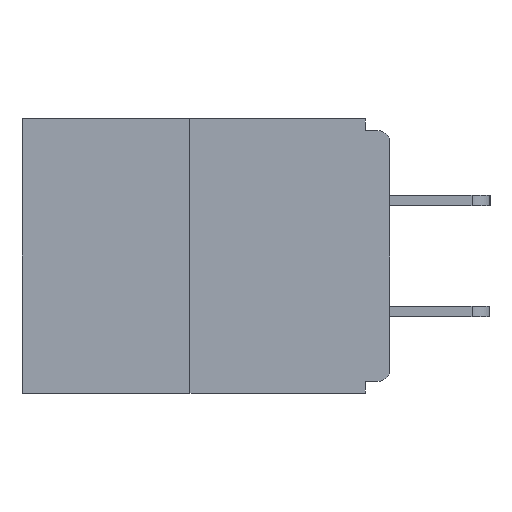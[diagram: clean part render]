
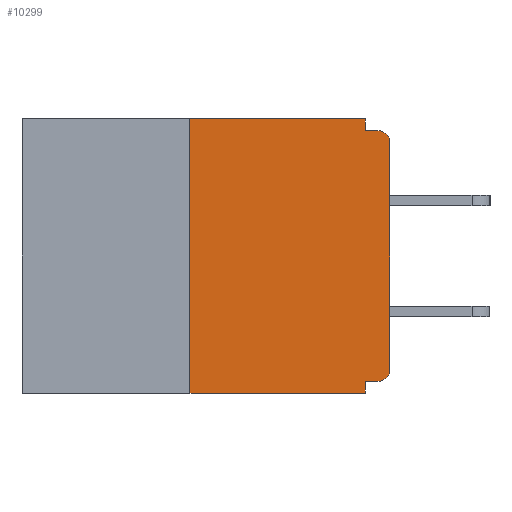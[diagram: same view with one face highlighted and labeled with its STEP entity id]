
A CAD part, left-side view. The second image highlights one B-rep face of the part: STEP entity #10299.
In plain terms, the highlighted planar face has unit normal (-1, 0, 0).
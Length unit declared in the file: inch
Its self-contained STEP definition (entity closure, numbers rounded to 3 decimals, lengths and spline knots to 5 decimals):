
#517 = LINE ( 'NONE', #9732, #7745 ) ;
#551 = VERTEX_POINT ( 'NONE', #4970 ) ;
#664 = EDGE_CURVE ( 'NONE', #4045, #1110, #4424, .T. ) ;
#794 = VERTEX_POINT ( 'NONE', #8882 ) ;
#1110 = VERTEX_POINT ( 'NONE', #6751 ) ;
#1453 = DIRECTION ( 'NONE',  ( 0., 0., -1. ) ) ;
#1519 = EDGE_LOOP ( 'NONE', ( #9037, #9609, #8001, #7870, #8754, #4073, #1643, #8099, #3055, #11710 ) ) ;
#1613 = VECTOR ( 'NONE', #11980, 39.37008 ) ;
#1643 = ORIENTED_EDGE ( 'NONE', *, *, #7530, .T. ) ;
#1729 = CARTESIAN_POINT ( 'NONE',  ( 0., 0., -0.328 ) ) ;
#1971 = EDGE_CURVE ( 'NONE', #551, #1110, #7246, .T. ) ;
#2063 = CARTESIAN_POINT ( 'NONE',  ( 0., 0.25, -0.343 ) ) ;
#2077 = CARTESIAN_POINT ( 'NONE',  ( 0., 0.46, 0. ) ) ;
#2398 = CARTESIAN_POINT ( 'NONE',  ( 0., 0.015, -0.313 ) ) ;
#2676 = CARTESIAN_POINT ( 'NONE',  ( 0., 0., -0.015 ) ) ;
#2871 = DIRECTION ( 'NONE',  ( 0., 0., -1. ) ) ;
#3010 = DIRECTION ( 'NONE',  ( 0., -1., 0. ) ) ;
#3019 = VERTEX_POINT ( 'NONE', #5567 ) ;
#3055 = ORIENTED_EDGE ( 'NONE', *, *, #1971, .F. ) ;
#3184 = LINE ( 'NONE', #6587, #3759 ) ;
#3208 = DIRECTION ( 'NONE',  ( 0., -1., 0. ) ) ;
#3209 = EDGE_CURVE ( 'NONE', #11686, #3019, #10383, .T. ) ;
#3398 = DIRECTION ( 'NONE',  ( 0., 0., -1. ) ) ;
#3759 = VECTOR ( 'NONE', #7569, 39.37008 ) ;
#3809 = CARTESIAN_POINT ( 'NONE',  ( 0., 0.015, -0.03 ) ) ;
#4045 = VERTEX_POINT ( 'NONE', #6718 ) ;
#4073 = ORIENTED_EDGE ( 'NONE', *, *, #4259, .T. ) ;
#4138 = LINE ( 'NONE', #10621, #4411 ) ;
#4259 = EDGE_CURVE ( 'NONE', #7593, #794, #4943, .T. ) ;
#4411 = VECTOR ( 'NONE', #3208, 39.37008 ) ;
#4424 = CIRCLE ( 'NONE', #7054, 0.015 ) ;
#4533 = EDGE_CURVE ( 'NONE', #8443, #11686, #8022, .T. ) ;
#4943 = CIRCLE ( 'NONE', #10012, 0.015 ) ;
#4970 = CARTESIAN_POINT ( 'NONE',  ( 0., 0.031, -0.015 ) ) ;
#5286 = CARTESIAN_POINT ( 'NONE',  ( 0., 0.25, 0. ) ) ;
#5435 = VECTOR ( 'NONE', #3010, 39.37008 ) ;
#5525 = DIRECTION ( 'NONE',  ( 0., 0., -1. ) ) ;
#5567 = CARTESIAN_POINT ( 'NONE',  ( 0., 0.031, 0. ) ) ;
#6142 = VECTOR ( 'NONE', #10893, 39.37008 ) ;
#6214 = VECTOR ( 'NONE', #9377, 39.37008 ) ;
#6487 = PLANE ( 'NONE',  #7070 ) ;
#6587 = CARTESIAN_POINT ( 'NONE',  ( 0., 0., 0. ) ) ;
#6595 = EDGE_CURVE ( 'NONE', #3019, #551, #517, .T. ) ;
#6718 = CARTESIAN_POINT ( 'NONE',  ( 0., 0., -0.03 ) ) ;
#6751 = CARTESIAN_POINT ( 'NONE',  ( 0., 0.015, -0.015 ) ) ;
#7054 = AXIS2_PLACEMENT_3D ( 'NONE', #3809, #8466, #2871 ) ;
#7070 = AXIS2_PLACEMENT_3D ( 'NONE', #10211, #8473, #7387 ) ;
#7149 = VERTEX_POINT ( 'NONE', #10819 ) ;
#7246 = LINE ( 'NONE', #2676, #6214 ) ;
#7387 = DIRECTION ( 'NONE',  ( 0., 0., -1. ) ) ;
#7530 = EDGE_CURVE ( 'NONE', #794, #4045, #3184, .T. ) ;
#7569 = DIRECTION ( 'NONE',  ( 0., 0., 1. ) ) ;
#7593 = VERTEX_POINT ( 'NONE', #9415 ) ;
#7745 = VECTOR ( 'NONE', #1453, 39.37008 ) ;
#7799 = VECTOR ( 'NONE', #5525, 39.37008 ) ;
#7870 = ORIENTED_EDGE ( 'NONE', *, *, #10167, .F. ) ;
#8001 = ORIENTED_EDGE ( 'NONE', *, *, #10001, .T. ) ;
#8022 = LINE ( 'NONE', #5286, #6142 ) ;
#8099 = ORIENTED_EDGE ( 'NONE', *, *, #664, .T. ) ;
#8350 = CARTESIAN_POINT ( 'NONE',  ( 0., 0.25, 0. ) ) ;
#8443 = VERTEX_POINT ( 'NONE', #2063 ) ;
#8466 = DIRECTION ( 'NONE',  ( -1., 0., 0. ) ) ;
#8473 = DIRECTION ( 'NONE',  ( 1., 0., 0. ) ) ;
#8754 = ORIENTED_EDGE ( 'NONE', *, *, #11629, .F. ) ;
#8882 = CARTESIAN_POINT ( 'NONE',  ( 0., 0., -0.313 ) ) ;
#9037 = ORIENTED_EDGE ( 'NONE', *, *, #3209, .F. ) ;
#9305 = VERTEX_POINT ( 'NONE', #11431 ) ;
#9377 = DIRECTION ( 'NONE',  ( 0., -1., 0. ) ) ;
#9415 = CARTESIAN_POINT ( 'NONE',  ( 0., 0.015, -0.328 ) ) ;
#9609 = ORIENTED_EDGE ( 'NONE', *, *, #4533, .F. ) ;
#9732 = CARTESIAN_POINT ( 'NONE',  ( 0., 0.031, 0. ) ) ;
#10001 = EDGE_CURVE ( 'NONE', #8443, #9305, #4138, .T. ) ;
#10012 = AXIS2_PLACEMENT_3D ( 'NONE', #2398, #10809, #3398 ) ;
#10167 = EDGE_CURVE ( 'NONE', #7149, #9305, #12004, .T. ) ;
#10211 = CARTESIAN_POINT ( 'NONE',  ( 0., 0.46, 0. ) ) ;
#10299 = ADVANCED_FACE ( 'NONE', ( #10553 ), #6487, .F. ) ;
#10383 = LINE ( 'NONE', #2077, #5435 ) ;
#10553 = FACE_OUTER_BOUND ( 'NONE', #1519, .T. ) ;
#10621 = CARTESIAN_POINT ( 'NONE',  ( 0., 0.46, -0.343 ) ) ;
#10809 = DIRECTION ( 'NONE',  ( -1., 0., 0. ) ) ;
#10819 = CARTESIAN_POINT ( 'NONE',  ( 0., 0.031, -0.328 ) ) ;
#10893 = DIRECTION ( 'NONE',  ( 0., 0., 1. ) ) ;
#11117 = CARTESIAN_POINT ( 'NONE',  ( 0., 0.031, -0.343 ) ) ;
#11431 = CARTESIAN_POINT ( 'NONE',  ( 0., 0.031, -0.343 ) ) ;
#11629 = EDGE_CURVE ( 'NONE', #7593, #7149, #12134, .T. ) ;
#11686 = VERTEX_POINT ( 'NONE', #8350 ) ;
#11710 = ORIENTED_EDGE ( 'NONE', *, *, #6595, .F. ) ;
#11980 = DIRECTION ( 'NONE',  ( 0., 1., 0. ) ) ;
#12004 = LINE ( 'NONE', #11117, #7799 ) ;
#12134 = LINE ( 'NONE', #1729, #1613 ) ;
